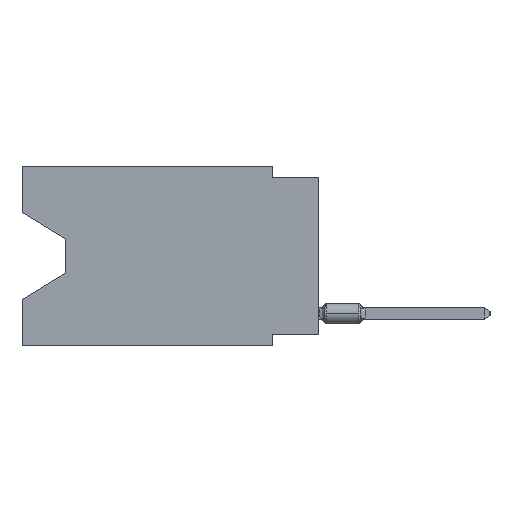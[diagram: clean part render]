
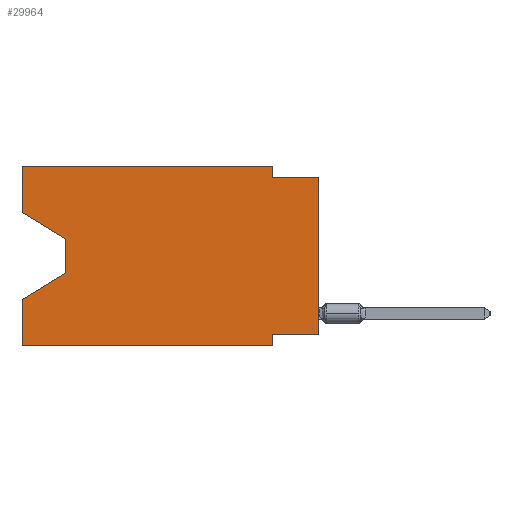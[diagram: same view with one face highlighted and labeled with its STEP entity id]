
A CAD part, left-side view. The second image highlights one B-rep face of the part: STEP entity #29964.
In plain terms, the highlighted planar face has unit normal (-1, 0, 0).
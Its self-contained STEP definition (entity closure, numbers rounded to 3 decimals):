
#27 = EDGE_CURVE ( 'NONE', #29439, #15707, #16515, .T. ) ;
#157 = ORIENTED_EDGE ( 'NONE', *, *, #10126, .T. ) ;
#256 = CARTESIAN_POINT ( 'NONE',  ( 0., 16.383, 0. ) ) ;
#684 = CARTESIAN_POINT ( 'NONE',  ( 0., 2.54, -9.906 ) ) ;
#1210 = VECTOR ( 'NONE', #26593, 1000. ) ;
#1275 = DIRECTION ( 'NONE',  ( 0., 0., 1. ) ) ;
#1340 = LINE ( 'NONE', #9602, #31810 ) ;
#1840 = CARTESIAN_POINT ( 'NONE',  ( 0., 2.54, 0. ) ) ;
#1953 = VECTOR ( 'NONE', #9584, 1000. ) ;
#2582 = ORIENTED_EDGE ( 'NONE', *, *, #12961, .F. ) ;
#2700 = ORIENTED_EDGE ( 'NONE', *, *, #34211, .F. ) ;
#3181 = LINE ( 'NONE', #17065, #1210 ) ;
#3304 = VECTOR ( 'NONE', #16985, 1000. ) ;
#3605 = CARTESIAN_POINT ( 'NONE',  ( 0., 13.97, -5.893 ) ) ;
#3954 = CARTESIAN_POINT ( 'NONE',  ( 0., 16.383, 0. ) ) ;
#4136 = PLANE ( 'NONE',  #33994 ) ;
#4578 = VERTEX_POINT ( 'NONE', #3605 ) ;
#5507 = VERTEX_POINT ( 'NONE', #29814 ) ;
#6257 = CARTESIAN_POINT ( 'NONE',  ( 0., 0., -0.635 ) ) ;
#7572 = CARTESIAN_POINT ( 'NONE',  ( 0., 2.54, -9.271 ) ) ;
#7682 = DIRECTION ( 'NONE',  ( 0., 0., 1. ) ) ;
#8232 = ORIENTED_EDGE ( 'NONE', *, *, #10051, .F. ) ;
#8799 = CARTESIAN_POINT ( 'NONE',  ( 0., 16.383, -2.546 ) ) ;
#9313 = VECTOR ( 'NONE', #34673, 1000. ) ;
#9422 = DIRECTION ( 'NONE',  ( 0., 0., -1. ) ) ;
#9584 = DIRECTION ( 'NONE',  ( 0., 0., -1. ) ) ;
#9602 = CARTESIAN_POINT ( 'NONE',  ( 0., 13.97, -5.893 ) ) ;
#9777 = EDGE_CURVE ( 'NONE', #26947, #29225, #10815, .T. ) ;
#9897 = VECTOR ( 'NONE', #30040, 1000. ) ;
#10051 = EDGE_CURVE ( 'NONE', #19226, #12849, #33621, .T. ) ;
#10126 = EDGE_CURVE ( 'NONE', #26947, #27104, #24970, .T. ) ;
#10288 = VECTOR ( 'NONE', #34584, 1000. ) ;
#10511 = LINE ( 'NONE', #29464, #24980 ) ;
#10815 = LINE ( 'NONE', #256, #9313 ) ;
#11044 = CARTESIAN_POINT ( 'NONE',  ( 0., 16.383, -9.906 ) ) ;
#11089 = VECTOR ( 'NONE', #32995, 1000. ) ;
#11328 = CARTESIAN_POINT ( 'NONE',  ( 0., 16.383, 0. ) ) ;
#11699 = DIRECTION ( 'NONE',  ( 1., 0., 0. ) ) ;
#11892 = DIRECTION ( 'NONE',  ( 0., 0.855, -0.519 ) ) ;
#12377 = EDGE_LOOP ( 'NONE', ( #157, #20209, #12548, #22544, #31797, #16396, #2700, #18326, #2582, #8232, #14075, #16707 ) ) ;
#12548 = ORIENTED_EDGE ( 'NONE', *, *, #28414, .T. ) ;
#12590 = VECTOR ( 'NONE', #7682, 1000. ) ;
#12849 = VERTEX_POINT ( 'NONE', #14359 ) ;
#12961 = EDGE_CURVE ( 'NONE', #12849, #16513, #30307, .T. ) ;
#13104 = EDGE_CURVE ( 'NONE', #29225, #19226, #29927, .T. ) ;
#13995 = VECTOR ( 'NONE', #27303, 1000. ) ;
#14075 = ORIENTED_EDGE ( 'NONE', *, *, #13104, .F. ) ;
#14346 = CARTESIAN_POINT ( 'NONE',  ( 0., 13.97, -4.013 ) ) ;
#14359 = CARTESIAN_POINT ( 'NONE',  ( 0., 2.54, -0.635 ) ) ;
#14632 = LINE ( 'NONE', #22532, #32678 ) ;
#14799 = VERTEX_POINT ( 'NONE', #11044 ) ;
#15510 = EDGE_CURVE ( 'NONE', #14799, #15707, #3181, .T. ) ;
#15628 = CARTESIAN_POINT ( 'NONE',  ( 0., 0., -0.635 ) ) ;
#15707 = VERTEX_POINT ( 'NONE', #17413 ) ;
#16396 = ORIENTED_EDGE ( 'NONE', *, *, #27, .F. ) ;
#16513 = VERTEX_POINT ( 'NONE', #15628 ) ;
#16515 = LINE ( 'NONE', #684, #11089 ) ;
#16707 = ORIENTED_EDGE ( 'NONE', *, *, #9777, .F. ) ;
#16985 = DIRECTION ( 'NONE',  ( 0., -1., 0. ) ) ;
#17065 = CARTESIAN_POINT ( 'NONE',  ( 0., 16.383, -9.906 ) ) ;
#17413 = CARTESIAN_POINT ( 'NONE',  ( 0., 2.54, -9.906 ) ) ;
#17903 = EDGE_CURVE ( 'NONE', #27104, #4578, #26694, .T. ) ;
#18326 = ORIENTED_EDGE ( 'NONE', *, *, #18355, .T. ) ;
#18355 = EDGE_CURVE ( 'NONE', #19909, #16513, #26479, .T. ) ;
#19226 = VERTEX_POINT ( 'NONE', #27025 ) ;
#19909 = VERTEX_POINT ( 'NONE', #34458 ) ;
#20209 = ORIENTED_EDGE ( 'NONE', *, *, #17903, .T. ) ;
#21048 = CARTESIAN_POINT ( 'NONE',  ( 0., 0., 0. ) ) ;
#22532 = CARTESIAN_POINT ( 'NONE',  ( 0., 16.383, 0. ) ) ;
#22544 = ORIENTED_EDGE ( 'NONE', *, *, #23683, .F. ) ;
#23556 = CARTESIAN_POINT ( 'NONE',  ( 0., 13.97, -4.013 ) ) ;
#23683 = EDGE_CURVE ( 'NONE', #14799, #5507, #14632, .T. ) ;
#24970 = LINE ( 'NONE', #8799, #9897 ) ;
#24980 = VECTOR ( 'NONE', #31410, 1000. ) ;
#26479 = LINE ( 'NONE', #21048, #12590 ) ;
#26593 = DIRECTION ( 'NONE',  ( 0., -1., 0. ) ) ;
#26694 = LINE ( 'NONE', #23556, #10288 ) ;
#26947 = VERTEX_POINT ( 'NONE', #32052 ) ;
#27025 = CARTESIAN_POINT ( 'NONE',  ( 0., 2.54, 0. ) ) ;
#27104 = VERTEX_POINT ( 'NONE', #14346 ) ;
#27303 = DIRECTION ( 'NONE',  ( 0., -1., 0. ) ) ;
#28026 = FACE_OUTER_BOUND ( 'NONE', #12377, .T. ) ;
#28414 = EDGE_CURVE ( 'NONE', #4578, #5507, #1340, .T. ) ;
#29225 = VERTEX_POINT ( 'NONE', #32865 ) ;
#29439 = VERTEX_POINT ( 'NONE', #7572 ) ;
#29464 = CARTESIAN_POINT ( 'NONE',  ( 0., 0., -9.271 ) ) ;
#29814 = CARTESIAN_POINT ( 'NONE',  ( 0., 16.383, -7.36 ) ) ;
#29927 = LINE ( 'NONE', #11328, #13995 ) ;
#29964 = ADVANCED_FACE ( 'NONE', ( #28026 ), #4136, .F. ) ;
#30040 = DIRECTION ( 'NONE',  ( 0., -0.855, -0.519 ) ) ;
#30307 = LINE ( 'NONE', #6257, #3304 ) ;
#31410 = DIRECTION ( 'NONE',  ( 0., 1., 0. ) ) ;
#31797 = ORIENTED_EDGE ( 'NONE', *, *, #15510, .T. ) ;
#31810 = VECTOR ( 'NONE', #11892, 1000. ) ;
#32052 = CARTESIAN_POINT ( 'NONE',  ( 0., 16.383, -2.546 ) ) ;
#32678 = VECTOR ( 'NONE', #1275, 1000. ) ;
#32865 = CARTESIAN_POINT ( 'NONE',  ( 0., 16.383, 0. ) ) ;
#32995 = DIRECTION ( 'NONE',  ( 0., 0., -1. ) ) ;
#33621 = LINE ( 'NONE', #1840, #1953 ) ;
#33994 = AXIS2_PLACEMENT_3D ( 'NONE', #3954, #11699, #9422 ) ;
#34211 = EDGE_CURVE ( 'NONE', #19909, #29439, #10511, .T. ) ;
#34458 = CARTESIAN_POINT ( 'NONE',  ( 0., 0., -9.271 ) ) ;
#34584 = DIRECTION ( 'NONE',  ( 0., 0., -1. ) ) ;
#34673 = DIRECTION ( 'NONE',  ( 0., 0., 1. ) ) ;
